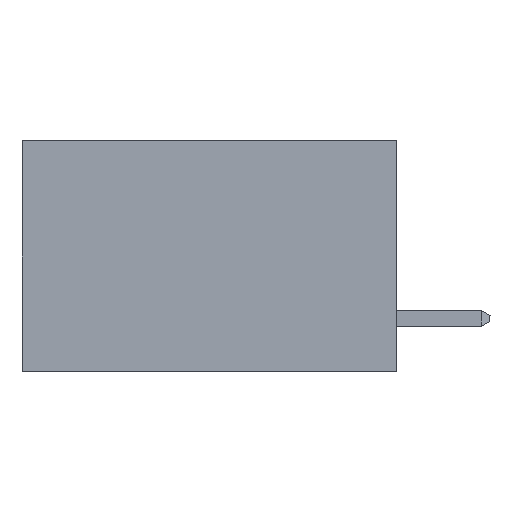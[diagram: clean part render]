
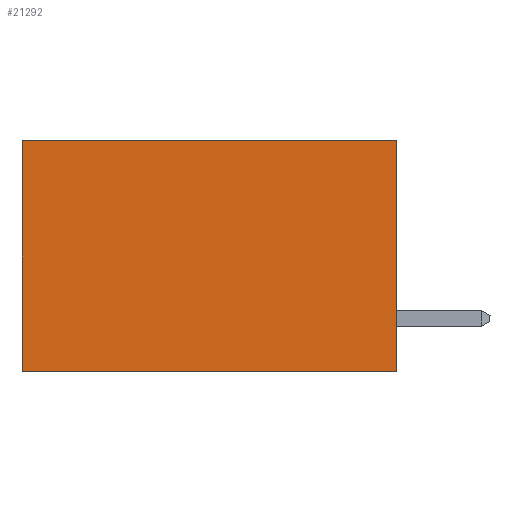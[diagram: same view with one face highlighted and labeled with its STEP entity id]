
A CAD part, left-side view. The second image highlights one B-rep face of the part: STEP entity #21292.
In plain terms, the highlighted planar face has unit normal (-1, 0, 0).
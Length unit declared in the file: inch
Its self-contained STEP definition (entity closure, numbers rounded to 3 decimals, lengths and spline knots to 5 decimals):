
#261 = LINE ( 'NONE', #10098, #882 ) ;
#659 = DIRECTION ( 'NONE',  ( 0., 1., 0. ) ) ;
#882 = VECTOR ( 'NONE', #8155, 39.37008 ) ;
#1257 = AXIS2_PLACEMENT_3D ( 'NONE', #6736, #4678, #1376 ) ;
#1376 = DIRECTION ( 'NONE',  ( 0., 0., -1. ) ) ;
#2553 = VECTOR ( 'NONE', #5344, 39.37008 ) ;
#2985 = CARTESIAN_POINT ( 'NONE',  ( 0.2615, 0., 0. ) ) ;
#4178 = CARTESIAN_POINT ( 'NONE',  ( 0.2615, 0., -0.37 ) ) ;
#4678 = DIRECTION ( 'NONE',  ( 1., 0., 0. ) ) ;
#5330 = VERTEX_POINT ( 'NONE', #17998 ) ;
#5344 = DIRECTION ( 'NONE',  ( 0., 0., -1. ) ) ;
#5365 = LINE ( 'NONE', #7559, #18735 ) ;
#6133 = VERTEX_POINT ( 'NONE', #2985 ) ;
#6736 = CARTESIAN_POINT ( 'NONE',  ( 0.2615, 0., -0.37 ) ) ;
#7559 = CARTESIAN_POINT ( 'NONE',  ( 0.2615, 0., -0.37 ) ) ;
#8155 = DIRECTION ( 'NONE',  ( 0., 1., 0. ) ) ;
#8466 = EDGE_CURVE ( 'NONE', #11026, #5330, #23783, .T. ) ;
#10098 = CARTESIAN_POINT ( 'NONE',  ( 0.2615, 0., 0. ) ) ;
#11026 = VERTEX_POINT ( 'NONE', #13646 ) ;
#12002 = ORIENTED_EDGE ( 'NONE', *, *, #18115, .F. ) ;
#12198 = ORIENTED_EDGE ( 'NONE', *, *, #21833, .T. ) ;
#12794 = VECTOR ( 'NONE', #659, 39.37008 ) ;
#13646 = CARTESIAN_POINT ( 'NONE',  ( 0.2615, 0.6, 0. ) ) ;
#14575 = CARTESIAN_POINT ( 'NONE',  ( 0.2615, 0.6, -0.37 ) ) ;
#17177 = CARTESIAN_POINT ( 'NONE',  ( 0.2615, 0., -0.37 ) ) ;
#17228 = ORIENTED_EDGE ( 'NONE', *, *, #21756, .F. ) ;
#17544 = LINE ( 'NONE', #17177, #12794 ) ;
#17671 = PLANE ( 'NONE',  #1257 ) ;
#17998 = CARTESIAN_POINT ( 'NONE',  ( 0.2615, 0.6, -0.37 ) ) ;
#18115 = EDGE_CURVE ( 'NONE', #22808, #5330, #17544, .T. ) ;
#18735 = VECTOR ( 'NONE', #20407, 39.37008 ) ;
#19858 = ORIENTED_EDGE ( 'NONE', *, *, #8466, .T. ) ;
#20407 = DIRECTION ( 'NONE',  ( 0., 0., -1. ) ) ;
#21290 = FACE_OUTER_BOUND ( 'NONE', #23112, .T. ) ;
#21292 = ADVANCED_FACE ( 'NONE', ( #21290 ), #17671, .F. ) ;
#21756 = EDGE_CURVE ( 'NONE', #6133, #22808, #5365, .T. ) ;
#21833 = EDGE_CURVE ( 'NONE', #6133, #11026, #261, .T. ) ;
#22808 = VERTEX_POINT ( 'NONE', #4178 ) ;
#23112 = EDGE_LOOP ( 'NONE', ( #19858, #12002, #17228, #12198 ) ) ;
#23783 = LINE ( 'NONE', #14575, #2553 ) ;
